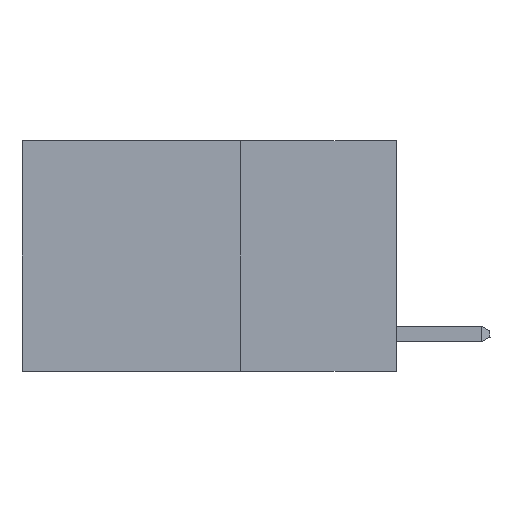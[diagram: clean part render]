
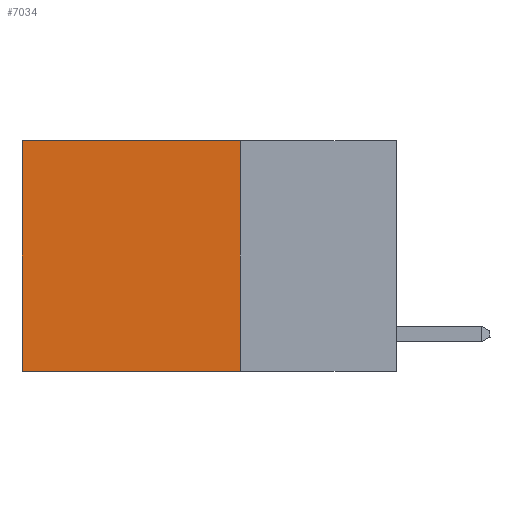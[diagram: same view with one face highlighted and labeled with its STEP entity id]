
A CAD part, left-side view. The second image highlights one B-rep face of the part: STEP entity #7034.
In plain terms, the highlighted planar face has unit normal (-1, 0, 0).
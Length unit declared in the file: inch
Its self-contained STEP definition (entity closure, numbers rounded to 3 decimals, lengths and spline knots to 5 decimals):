
#118 = VECTOR ( 'NONE', #2685, 39.37008 ) ;
#389 = EDGE_CURVE ( 'NONE', #641, #8871, #4795, .T. ) ;
#530 = CARTESIAN_POINT ( 'NONE',  ( 0.2625, 0.25, 0. ) ) ;
#641 = VERTEX_POINT ( 'NONE', #9581 ) ;
#968 = ORIENTED_EDGE ( 'NONE', *, *, #5214, .F. ) ;
#1373 = DIRECTION ( 'NONE',  ( 0., 0., -1. ) ) ;
#1457 = LINE ( 'NONE', #11003, #8671 ) ;
#2685 = DIRECTION ( 'NONE',  ( 0., 1., 0. ) ) ;
#2922 = EDGE_CURVE ( 'NONE', #5117, #641, #1457, .T. ) ;
#3840 = ORIENTED_EDGE ( 'NONE', *, *, #2922, .T. ) ;
#4023 = CARTESIAN_POINT ( 'NONE',  ( 0.2625, 0.6, 0. ) ) ;
#4560 = CARTESIAN_POINT ( 'NONE',  ( 0.2625, 0.25, -0.37 ) ) ;
#4607 = CARTESIAN_POINT ( 'NONE',  ( 0.2625, 0.25, 0. ) ) ;
#4727 = DIRECTION ( 'NONE',  ( 0., 0., -1. ) ) ;
#4795 = LINE ( 'NONE', #4023, #6681 ) ;
#5002 = VECTOR ( 'NONE', #4727, 39.37008 ) ;
#5117 = VERTEX_POINT ( 'NONE', #530 ) ;
#5143 = VERTEX_POINT ( 'NONE', #10071 ) ;
#5214 = EDGE_CURVE ( 'NONE', #5143, #8871, #9892, .T. ) ;
#5543 = DIRECTION ( 'NONE',  ( 1., 0., 0. ) ) ;
#6681 = VECTOR ( 'NONE', #1373, 39.37008 ) ;
#7034 = ADVANCED_FACE ( 'NONE', ( #7657 ), #11120, .F. ) ;
#7657 = FACE_OUTER_BOUND ( 'NONE', #10418, .T. ) ;
#7781 = LINE ( 'NONE', #11237, #5002 ) ;
#8323 = EDGE_CURVE ( 'NONE', #5117, #5143, #7781, .T. ) ;
#8509 = ORIENTED_EDGE ( 'NONE', *, *, #8323, .F. ) ;
#8671 = VECTOR ( 'NONE', #9141, 39.37008 ) ;
#8871 = VERTEX_POINT ( 'NONE', #9336 ) ;
#9141 = DIRECTION ( 'NONE',  ( 0., 1., 0. ) ) ;
#9285 = AXIS2_PLACEMENT_3D ( 'NONE', #4607, #5543, #12062 ) ;
#9336 = CARTESIAN_POINT ( 'NONE',  ( 0.2625, 0.6, -0.37 ) ) ;
#9581 = CARTESIAN_POINT ( 'NONE',  ( 0.2625, 0.6, 0. ) ) ;
#9892 = LINE ( 'NONE', #4560, #118 ) ;
#10071 = CARTESIAN_POINT ( 'NONE',  ( 0.2625, 0.25, -0.37 ) ) ;
#10418 = EDGE_LOOP ( 'NONE', ( #10700, #968, #8509, #3840 ) ) ;
#10700 = ORIENTED_EDGE ( 'NONE', *, *, #389, .T. ) ;
#11003 = CARTESIAN_POINT ( 'NONE',  ( 0.2625, 0.25, 0. ) ) ;
#11120 = PLANE ( 'NONE',  #9285 ) ;
#11237 = CARTESIAN_POINT ( 'NONE',  ( 0.2625, 0.25, 0. ) ) ;
#12062 = DIRECTION ( 'NONE',  ( 0., 0., -1. ) ) ;
